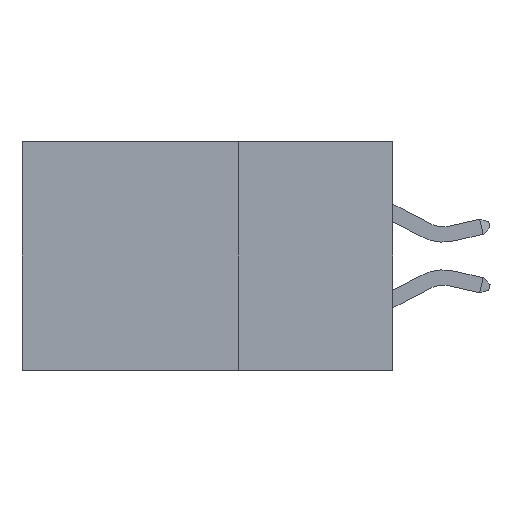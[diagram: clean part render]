
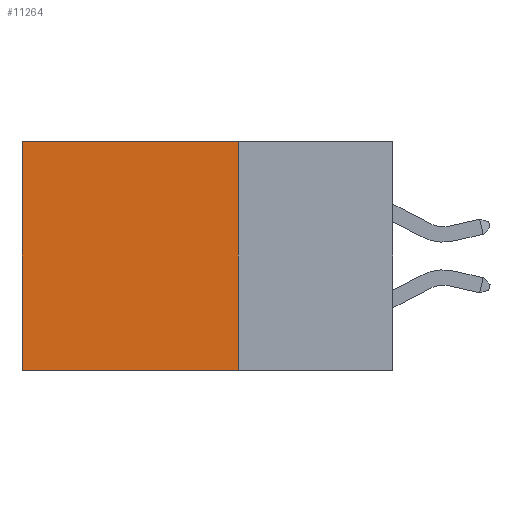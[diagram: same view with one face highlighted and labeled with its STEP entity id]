
A CAD part, left-side view. The second image highlights one B-rep face of the part: STEP entity #11264.
In plain terms, the highlighted planar face has unit normal (-1, 0, 0).
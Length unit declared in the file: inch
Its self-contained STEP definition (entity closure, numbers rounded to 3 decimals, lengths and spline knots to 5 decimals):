
#1 = LINE ( 'NONE', #4463, #558 ) ;
#485 = CARTESIAN_POINT ( 'NONE',  ( 0.2875, 0.6, 0. ) ) ;
#558 = VECTOR ( 'NONE', #9301, 39.37008 ) ;
#587 = PLANE ( 'NONE',  #10767 ) ;
#1660 = DIRECTION ( 'NONE',  ( 0., 0., -1. ) ) ;
#1951 = FACE_OUTER_BOUND ( 'NONE', #6246, .T. ) ;
#2492 = ORIENTED_EDGE ( 'NONE', *, *, #4089, .F. ) ;
#2631 = CARTESIAN_POINT ( 'NONE',  ( 0.2875, 0.25, 0. ) ) ;
#2962 = CARTESIAN_POINT ( 'NONE',  ( 0.2875, 0.25, 0. ) ) ;
#3138 = CARTESIAN_POINT ( 'NONE',  ( 0.2875, 0.25, -0.37 ) ) ;
#3734 = EDGE_CURVE ( 'NONE', #3850, #8294, #5827, .T. ) ;
#3850 = VERTEX_POINT ( 'NONE', #12371 ) ;
#4061 = DIRECTION ( 'NONE',  ( 0., 0., -1. ) ) ;
#4066 = ORIENTED_EDGE ( 'NONE', *, *, #11489, .F. ) ;
#4089 = EDGE_CURVE ( 'NONE', #15456, #15022, #1, .T. ) ;
#4463 = CARTESIAN_POINT ( 'NONE',  ( 0.2875, 0.25, -0.37 ) ) ;
#4511 = ORIENTED_EDGE ( 'NONE', *, *, #15054, .T. ) ;
#4961 = VECTOR ( 'NONE', #1660, 39.37008 ) ;
#5302 = DIRECTION ( 'NONE',  ( 1., 0., 0. ) ) ;
#5827 = LINE ( 'NONE', #2631, #6225 ) ;
#5872 = CARTESIAN_POINT ( 'NONE',  ( 0.2875, 0.6, 0. ) ) ;
#6225 = VECTOR ( 'NONE', #12235, 39.37008 ) ;
#6246 = EDGE_LOOP ( 'NONE', ( #4511, #2492, #4066, #9365 ) ) ;
#6283 = LINE ( 'NONE', #485, #12265 ) ;
#7486 = CARTESIAN_POINT ( 'NONE',  ( 0.2875, 0.25, 0. ) ) ;
#7594 = LINE ( 'NONE', #7486, #4961 ) ;
#8294 = VERTEX_POINT ( 'NONE', #5872 ) ;
#9301 = DIRECTION ( 'NONE',  ( 0., 1., 0. ) ) ;
#9365 = ORIENTED_EDGE ( 'NONE', *, *, #3734, .T. ) ;
#10311 = DIRECTION ( 'NONE',  ( 0., 0., -1. ) ) ;
#10767 = AXIS2_PLACEMENT_3D ( 'NONE', #2962, #5302, #10311 ) ;
#11201 = CARTESIAN_POINT ( 'NONE',  ( 0.2875, 0.6, -0.37 ) ) ;
#11264 = ADVANCED_FACE ( 'NONE', ( #1951 ), #587, .F. ) ;
#11489 = EDGE_CURVE ( 'NONE', #3850, #15456, #7594, .T. ) ;
#12235 = DIRECTION ( 'NONE',  ( 0., 1., 0. ) ) ;
#12265 = VECTOR ( 'NONE', #4061, 39.37008 ) ;
#12371 = CARTESIAN_POINT ( 'NONE',  ( 0.2875, 0.25, 0. ) ) ;
#15022 = VERTEX_POINT ( 'NONE', #11201 ) ;
#15054 = EDGE_CURVE ( 'NONE', #8294, #15022, #6283, .T. ) ;
#15456 = VERTEX_POINT ( 'NONE', #3138 ) ;
